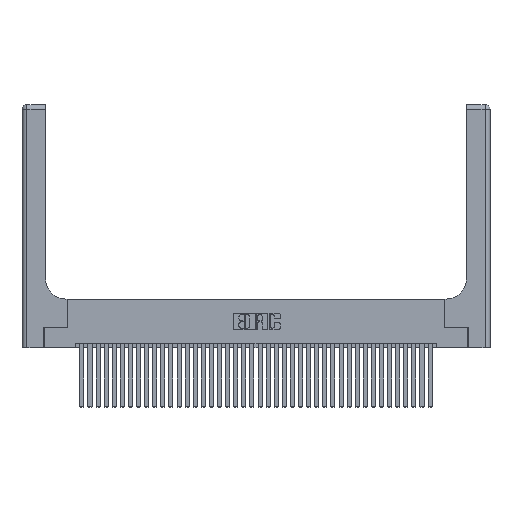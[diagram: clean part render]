
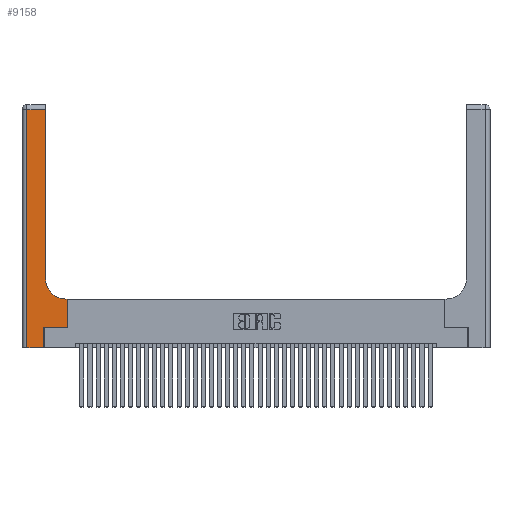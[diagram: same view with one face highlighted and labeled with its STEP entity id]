
A CAD part, top view. The second image highlights one B-rep face of the part: STEP entity #9158.
In plain terms, the highlighted planar face has unit normal (0, 0, 1).
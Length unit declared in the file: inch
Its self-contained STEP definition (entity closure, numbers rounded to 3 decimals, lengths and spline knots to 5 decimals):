
#301 = EDGE_CURVE ( 'NONE', #12398, #35562, #35085, .T. ) ;
#806 = CARTESIAN_POINT ( 'NONE',  ( 0.269, 0., 0.37 ) ) ;
#807 = CIRCLE ( 'NONE', #23447, 0.25 ) ;
#983 = ORIENTED_EDGE ( 'NONE', *, *, #37552, .T. ) ;
#2274 = CARTESIAN_POINT ( 'NONE',  ( 0.06, 2.94, 0.37 ) ) ;
#2395 = DIRECTION ( 'NONE',  ( 0., 0., -1. ) ) ;
#3257 = CARTESIAN_POINT ( 'NONE',  ( 0.269, 0., 0.37 ) ) ;
#3468 = CARTESIAN_POINT ( 'NONE',  ( 0.269, 0.25, 0.37 ) ) ;
#3686 = EDGE_CURVE ( 'NONE', #16827, #18576, #807, .T. ) ;
#3731 = CARTESIAN_POINT ( 'NONE',  ( 0.5415, 0.85, 0.37 ) ) ;
#4380 = CARTESIAN_POINT ( 'NONE',  ( 0.5585, 0.25, 0.37 ) ) ;
#5607 = CARTESIAN_POINT ( 'NONE',  ( 0.5415, 0.6, 0.37 ) ) ;
#5649 = EDGE_CURVE ( 'NONE', #12274, #18082, #23162, .T. ) ;
#6007 = VECTOR ( 'NONE', #28120, 39.37008 ) ;
#6140 = DIRECTION ( 'NONE',  ( -1., 0., 0. ) ) ;
#6343 = LINE ( 'NONE', #38264, #21584 ) ;
#6593 = LINE ( 'NONE', #10360, #13798 ) ;
#6864 = DIRECTION ( 'NONE',  ( 1., 0., 0. ) ) ;
#7142 = EDGE_CURVE ( 'NONE', #18576, #12398, #20200, .T. ) ;
#7529 = ORIENTED_EDGE ( 'NONE', *, *, #8402, .T. ) ;
#7950 = CARTESIAN_POINT ( 'NONE',  ( 0.06, 3., 0.37 ) ) ;
#8402 = EDGE_CURVE ( 'NONE', #15031, #18143, #18745, .T. ) ;
#9158 = ADVANCED_FACE ( 'NONE', ( #29434 ), #32893, .F. ) ;
#9655 = VECTOR ( 'NONE', #25668, 39.37008 ) ;
#10360 = CARTESIAN_POINT ( 'NONE',  ( 0.2915, 0.6, 0.37 ) ) ;
#10593 = LINE ( 'NONE', #13585, #9655 ) ;
#11203 = VERTEX_POINT ( 'NONE', #22960 ) ;
#11252 = LINE ( 'NONE', #7950, #20303 ) ;
#11439 = CARTESIAN_POINT ( 'NONE',  ( 0.2915, 3., 0.37 ) ) ;
#12056 = VECTOR ( 'NONE', #6140, 39.37008 ) ;
#12274 = VERTEX_POINT ( 'NONE', #3257 ) ;
#12398 = VERTEX_POINT ( 'NONE', #34470 ) ;
#13585 = CARTESIAN_POINT ( 'NONE',  ( 0.269, 0.25, 0.37 ) ) ;
#13798 = VECTOR ( 'NONE', #22575, 39.37008 ) ;
#13925 = DIRECTION ( 'NONE',  ( 0., 1., 0. ) ) ;
#14179 = ORIENTED_EDGE ( 'NONE', *, *, #31694, .T. ) ;
#14566 = DIRECTION ( 'NONE',  ( 0., 1., 0. ) ) ;
#14971 = DIRECTION ( 'NONE',  ( -1., 0., 0. ) ) ;
#15031 = VERTEX_POINT ( 'NONE', #4380 ) ;
#16827 = VERTEX_POINT ( 'NONE', #5607 ) ;
#17346 = DIRECTION ( 'NONE',  ( 1., 0., 0. ) ) ;
#18082 = VERTEX_POINT ( 'NONE', #3468 ) ;
#18143 = VERTEX_POINT ( 'NONE', #36924 ) ;
#18576 = VERTEX_POINT ( 'NONE', #38857 ) ;
#18745 = LINE ( 'NONE', #34759, #31821 ) ;
#20200 = LINE ( 'NONE', #11439, #27232 ) ;
#20303 = VECTOR ( 'NONE', #29094, 39.37008 ) ;
#20494 = ORIENTED_EDGE ( 'NONE', *, *, #7142, .T. ) ;
#21584 = VECTOR ( 'NONE', #17346, 39.37008 ) ;
#22508 = ORIENTED_EDGE ( 'NONE', *, *, #27691, .T. ) ;
#22575 = DIRECTION ( 'NONE',  ( -1., 0., 0. ) ) ;
#22960 = CARTESIAN_POINT ( 'NONE',  ( 0.06, 0., 0.37 ) ) ;
#23162 = LINE ( 'NONE', #806, #6007 ) ;
#23447 = AXIS2_PLACEMENT_3D ( 'NONE', #3731, #25043, #6864 ) ;
#25043 = DIRECTION ( 'NONE',  ( 0., 0., -1. ) ) ;
#25668 = DIRECTION ( 'NONE',  ( 1., 0., 0. ) ) ;
#25917 = ORIENTED_EDGE ( 'NONE', *, *, #3686, .T. ) ;
#27232 = VECTOR ( 'NONE', #14566, 39.37008 ) ;
#27355 = CARTESIAN_POINT ( 'NONE',  ( 0., 2.94, 0.37 ) ) ;
#27691 = EDGE_CURVE ( 'NONE', #11203, #12274, #6343, .T. ) ;
#28120 = DIRECTION ( 'NONE',  ( 0., 1., 0. ) ) ;
#28206 = EDGE_CURVE ( 'NONE', #18082, #15031, #10593, .T. ) ;
#28517 = AXIS2_PLACEMENT_3D ( 'NONE', #29911, #2395, #14971 ) ;
#29094 = DIRECTION ( 'NONE',  ( 0., -1., 0. ) ) ;
#29434 = FACE_OUTER_BOUND ( 'NONE', #34054, .T. ) ;
#29911 = CARTESIAN_POINT ( 'NONE',  ( 0., 3., 0.37 ) ) ;
#31694 = EDGE_CURVE ( 'NONE', #18143, #16827, #6593, .T. ) ;
#31821 = VECTOR ( 'NONE', #13925, 39.37008 ) ;
#32636 = ORIENTED_EDGE ( 'NONE', *, *, #5649, .T. ) ;
#32893 = PLANE ( 'NONE',  #28517 ) ;
#34054 = EDGE_LOOP ( 'NONE', ( #20494, #37486, #983, #22508, #32636, #35033, #7529, #14179, #25917 ) ) ;
#34470 = CARTESIAN_POINT ( 'NONE',  ( 0.2915, 2.94, 0.37 ) ) ;
#34759 = CARTESIAN_POINT ( 'NONE',  ( 0.5585, 0.25, 0.37 ) ) ;
#35033 = ORIENTED_EDGE ( 'NONE', *, *, #28206, .T. ) ;
#35085 = LINE ( 'NONE', #27355, #12056 ) ;
#35562 = VERTEX_POINT ( 'NONE', #2274 ) ;
#36924 = CARTESIAN_POINT ( 'NONE',  ( 0.5585, 0.6, 0.37 ) ) ;
#37486 = ORIENTED_EDGE ( 'NONE', *, *, #301, .T. ) ;
#37552 = EDGE_CURVE ( 'NONE', #35562, #11203, #11252, .T. ) ;
#38264 = CARTESIAN_POINT ( 'NONE',  ( 0., 0., 0.37 ) ) ;
#38857 = CARTESIAN_POINT ( 'NONE',  ( 0.2915, 0.85, 0.37 ) ) ;
